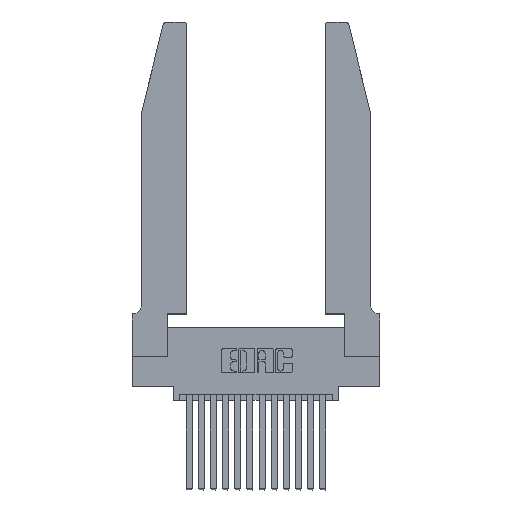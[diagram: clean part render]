
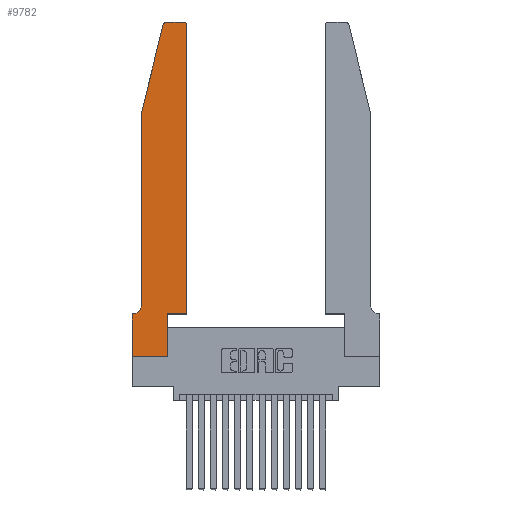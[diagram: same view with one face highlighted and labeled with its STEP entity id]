
A CAD part, top view. The second image highlights one B-rep face of the part: STEP entity #9782.
In plain terms, the highlighted planar face has unit normal (0, 0, 1).
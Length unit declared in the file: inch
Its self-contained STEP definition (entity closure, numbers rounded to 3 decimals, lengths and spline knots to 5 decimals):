
#232 = CARTESIAN_POINT ( 'NONE',  ( 0.284, 2.75, 0.37 ) ) ;
#342 = VECTOR ( 'NONE', #12005, 39.37008 ) ;
#792 = LINE ( 'NONE', #5226, #8491 ) ;
#795 = VECTOR ( 'NONE', #11231, 39.37008 ) ;
#909 = DIRECTION ( 'NONE',  ( -1., 0., 0. ) ) ;
#921 = ORIENTED_EDGE ( 'NONE', *, *, #17403, .T. ) ;
#975 = LINE ( 'NONE', #13739, #14643 ) ;
#1069 = EDGE_CURVE ( 'NONE', #14118, #9223, #10484, .T. ) ;
#1284 = CARTESIAN_POINT ( 'NONE',  ( 0.4505, 0.35, 0.37 ) ) ;
#1553 = VERTEX_POINT ( 'NONE', #9723 ) ;
#2055 = ORIENTED_EDGE ( 'NONE', *, *, #12408, .T. ) ;
#2085 = CARTESIAN_POINT ( 'NONE',  ( 0.25487, 2.72718, 0.37 ) ) ;
#2125 = VERTEX_POINT ( 'NONE', #8755 ) ;
#2154 = DIRECTION ( 'NONE',  ( 0., 1., 0. ) ) ;
#2165 = LINE ( 'NONE', #10691, #9316 ) ;
#2563 = EDGE_CURVE ( 'NONE', #1553, #2125, #17519, .T. ) ;
#2624 = VERTEX_POINT ( 'NONE', #11538 ) ;
#3162 = CARTESIAN_POINT ( 'NONE',  ( 0.0755, 2., 0.37 ) ) ;
#3231 = VERTEX_POINT ( 'NONE', #6554 ) ;
#3351 = ORIENTED_EDGE ( 'NONE', *, *, #1069, .T. ) ;
#3553 = ORIENTED_EDGE ( 'NONE', *, *, #2563, .T. ) ;
#3680 = DIRECTION ( 'NONE',  ( 0., -1., 0. ) ) ;
#3803 = LINE ( 'NONE', #1284, #795 ) ;
#4219 = EDGE_CURVE ( 'NONE', #5771, #9396, #3803, .T. ) ;
#4327 = ORIENTED_EDGE ( 'NONE', *, *, #4219, .T. ) ;
#4399 = CARTESIAN_POINT ( 'NONE',  ( 0.0055, 0.35, 0.37 ) ) ;
#4571 = EDGE_CURVE ( 'NONE', #14777, #1553, #2165, .T. ) ;
#4622 = DIRECTION ( 'NONE',  ( 0., -1., 0. ) ) ;
#4969 = VECTOR ( 'NONE', #4622, 39.37008 ) ;
#5121 = PLANE ( 'NONE',  #11801 ) ;
#5226 = CARTESIAN_POINT ( 'NONE',  ( 0.2605, 2.75, 0.37 ) ) ;
#5314 = EDGE_LOOP ( 'NONE', ( #17300, #10495, #15577, #921, #8433, #2055, #16149, #3553, #9715, #4327, #15946, #3351 ) ) ;
#5390 = CARTESIAN_POINT ( 'NONE',  ( 0.4505, 0.35, 0.37 ) ) ;
#5421 = CIRCLE ( 'NONE', #16112, 0.03 ) ;
#5528 = VERTEX_POINT ( 'NONE', #4399 ) ;
#5540 = CARTESIAN_POINT ( 'NONE',  ( 0.284, 2.72, 0.37 ) ) ;
#5613 = LINE ( 'NONE', #12060, #16176 ) ;
#5715 = CARTESIAN_POINT ( 'NONE',  ( 0.0755, 0.35, 0.37 ) ) ;
#5771 = VERTEX_POINT ( 'NONE', #14663 ) ;
#5909 = CIRCLE ( 'NONE', #12910, 0.07 ) ;
#6117 = DIRECTION ( 'NONE',  ( 1., 0., 0. ) ) ;
#6554 = CARTESIAN_POINT ( 'NONE',  ( 0.0755, 0.42, 0.37 ) ) ;
#6982 = DIRECTION ( 'NONE',  ( 1., 0., 0. ) ) ;
#7643 = CARTESIAN_POINT ( 'NONE',  ( 0., 0., 0.37 ) ) ;
#7805 = CARTESIAN_POINT ( 'NONE',  ( 0.4205, 2.72, 0.37 ) ) ;
#7988 = DIRECTION ( 'NONE',  ( 0., 0., 1. ) ) ;
#8068 = LINE ( 'NONE', #10608, #342 ) ;
#8433 = ORIENTED_EDGE ( 'NONE', *, *, #15998, .T. ) ;
#8491 = VECTOR ( 'NONE', #9332, 39.37008 ) ;
#8543 = DIRECTION ( 'NONE',  ( 0., 0., 1. ) ) ;
#8690 = VECTOR ( 'NONE', #14009, 39.37008 ) ;
#8740 = FACE_OUTER_BOUND ( 'NONE', #5314, .T. ) ;
#8755 = CARTESIAN_POINT ( 'NONE',  ( 0.2865, 0., 0.37 ) ) ;
#9223 = VERTEX_POINT ( 'NONE', #17394 ) ;
#9316 = VECTOR ( 'NONE', #3680, 39.37008 ) ;
#9332 = DIRECTION ( 'NONE',  ( -1., 0., 0. ) ) ;
#9396 = VERTEX_POINT ( 'NONE', #5390 ) ;
#9507 = DIRECTION ( 'NONE',  ( 0., 0., -1. ) ) ;
#9538 = LINE ( 'NONE', #5715, #8690 ) ;
#9715 = ORIENTED_EDGE ( 'NONE', *, *, #12132, .T. ) ;
#9723 = CARTESIAN_POINT ( 'NONE',  ( 0., 0., 0.37 ) ) ;
#9782 = ADVANCED_FACE ( 'NONE', ( #8740 ), #5121, .T. ) ;
#10484 = CIRCLE ( 'NONE', #17375, 0.03 ) ;
#10495 = ORIENTED_EDGE ( 'NONE', *, *, #17370, .T. ) ;
#10608 = CARTESIAN_POINT ( 'NONE',  ( 0.0755, 2., 0.37 ) ) ;
#10691 = CARTESIAN_POINT ( 'NONE',  ( 0., 0., 0.37 ) ) ;
#11231 = DIRECTION ( 'NONE',  ( 1., 0., 0. ) ) ;
#11365 = CARTESIAN_POINT ( 'NONE',  ( 0.4505, 2.72, 0.37 ) ) ;
#11370 = DIRECTION ( 'NONE',  ( 1., 0., 0. ) ) ;
#11538 = CARTESIAN_POINT ( 'NONE',  ( 0.0755, 2., 0.37 ) ) ;
#11801 = AXIS2_PLACEMENT_3D ( 'NONE', #16177, #7988, #17548 ) ;
#12005 = DIRECTION ( 'NONE',  ( -0.239, -0.971, 0. ) ) ;
#12019 = CARTESIAN_POINT ( 'NONE',  ( 0., 0.35, 0.37 ) ) ;
#12060 = CARTESIAN_POINT ( 'NONE',  ( 0.2865, 0.35, 0.37 ) ) ;
#12132 = EDGE_CURVE ( 'NONE', #2125, #5771, #5613, .T. ) ;
#12194 = EDGE_CURVE ( 'NONE', #9223, #17976, #792, .T. ) ;
#12408 = EDGE_CURVE ( 'NONE', #5528, #14777, #9538, .T. ) ;
#12910 = AXIS2_PLACEMENT_3D ( 'NONE', #17682, #9507, #909 ) ;
#13400 = EDGE_CURVE ( 'NONE', #9396, #14118, #975, .T. ) ;
#13739 = CARTESIAN_POINT ( 'NONE',  ( 0.4505, 0.35, 0.37 ) ) ;
#13881 = VERTEX_POINT ( 'NONE', #2085 ) ;
#14009 = DIRECTION ( 'NONE',  ( -1., 0., 0. ) ) ;
#14118 = VERTEX_POINT ( 'NONE', #11365 ) ;
#14308 = VECTOR ( 'NONE', #11370, 39.37008 ) ;
#14643 = VECTOR ( 'NONE', #15102, 39.37008 ) ;
#14663 = CARTESIAN_POINT ( 'NONE',  ( 0.2865, 0.35, 0.37 ) ) ;
#14777 = VERTEX_POINT ( 'NONE', #12019 ) ;
#15102 = DIRECTION ( 'NONE',  ( 0., 1., 0. ) ) ;
#15195 = DIRECTION ( 'NONE',  ( 0., 0., 1. ) ) ;
#15577 = ORIENTED_EDGE ( 'NONE', *, *, #18163, .T. ) ;
#15946 = ORIENTED_EDGE ( 'NONE', *, *, #13400, .T. ) ;
#15991 = LINE ( 'NONE', #3162, #4969 ) ;
#15998 = EDGE_CURVE ( 'NONE', #3231, #5528, #5909, .T. ) ;
#16112 = AXIS2_PLACEMENT_3D ( 'NONE', #5540, #15195, #6982 ) ;
#16149 = ORIENTED_EDGE ( 'NONE', *, *, #4571, .T. ) ;
#16176 = VECTOR ( 'NONE', #2154, 39.37008 ) ;
#16177 = CARTESIAN_POINT ( 'NONE',  ( 0., 0.35, 0.37 ) ) ;
#17300 = ORIENTED_EDGE ( 'NONE', *, *, #12194, .T. ) ;
#17370 = EDGE_CURVE ( 'NONE', #17976, #13881, #5421, .T. ) ;
#17375 = AXIS2_PLACEMENT_3D ( 'NONE', #7805, #8543, #6117 ) ;
#17394 = CARTESIAN_POINT ( 'NONE',  ( 0.4205, 2.75, 0.37 ) ) ;
#17403 = EDGE_CURVE ( 'NONE', #2624, #3231, #15991, .T. ) ;
#17519 = LINE ( 'NONE', #7643, #14308 ) ;
#17548 = DIRECTION ( 'NONE',  ( 1., 0., 0. ) ) ;
#17682 = CARTESIAN_POINT ( 'NONE',  ( 0.0055, 0.42, 0.37 ) ) ;
#17976 = VERTEX_POINT ( 'NONE', #232 ) ;
#18163 = EDGE_CURVE ( 'NONE', #13881, #2624, #8068, .T. ) ;
